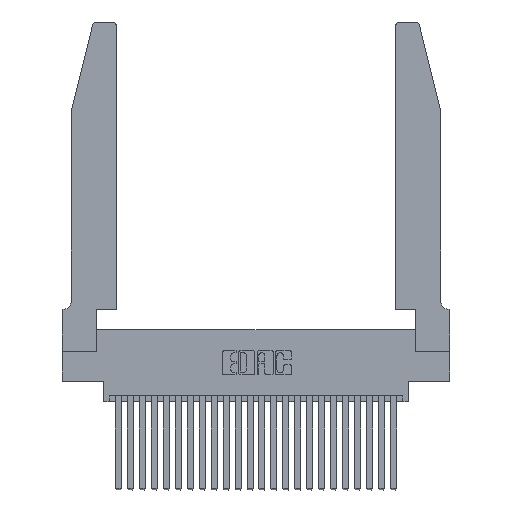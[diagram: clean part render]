
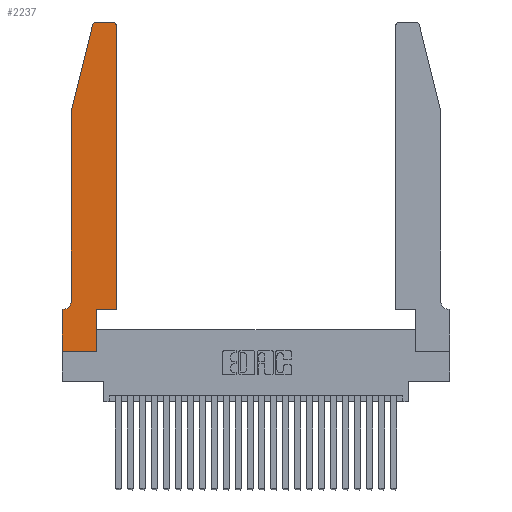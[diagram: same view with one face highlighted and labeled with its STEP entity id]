
A CAD part, top view. The second image highlights one B-rep face of the part: STEP entity #2237.
In plain terms, the highlighted planar face has unit normal (0, 0, 1).
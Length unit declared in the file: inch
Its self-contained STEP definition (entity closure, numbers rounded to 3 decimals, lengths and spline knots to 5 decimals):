
#209 = DIRECTION ( 'NONE',  ( 0., -1., 0. ) ) ;
#826 = PLANE ( 'NONE',  #3840 ) ;
#940 = DIRECTION ( 'NONE',  ( 1., 0., 0. ) ) ;
#1309 = VECTOR ( 'NONE', #20202, 39.37008 ) ;
#1359 = ORIENTED_EDGE ( 'NONE', *, *, #10340, .T. ) ;
#1753 = CARTESIAN_POINT ( 'NONE',  ( 0., 0.35, 0.37 ) ) ;
#2237 = ADVANCED_FACE ( 'NONE', ( #5001 ), #826, .T. ) ;
#2277 = DIRECTION ( 'NONE',  ( 0., 0., -1. ) ) ;
#2393 = AXIS2_PLACEMENT_3D ( 'NONE', #6460, #20418, #8505 ) ;
#2628 = EDGE_CURVE ( 'NONE', #16417, #22275, #22827, .T. ) ;
#2946 = EDGE_CURVE ( 'NONE', #23687, #5121, #10706, .T. ) ;
#3197 = CARTESIAN_POINT ( 'NONE',  ( 0., 0., 0.37 ) ) ;
#3604 = EDGE_CURVE ( 'NONE', #17030, #17161, #9738, .T. ) ;
#3840 = AXIS2_PLACEMENT_3D ( 'NONE', #1753, #6134, #940 ) ;
#3961 = VERTEX_POINT ( 'NONE', #18576 ) ;
#4518 = CIRCLE ( 'NONE', #2393, 0.03 ) ;
#4694 = CARTESIAN_POINT ( 'NONE',  ( 0.0055, 0.35, 0.37 ) ) ;
#5001 = FACE_OUTER_BOUND ( 'NONE', #18183, .T. ) ;
#5083 = VERTEX_POINT ( 'NONE', #9892 ) ;
#5121 = VERTEX_POINT ( 'NONE', #12223 ) ;
#6134 = DIRECTION ( 'NONE',  ( 0., 0., 1. ) ) ;
#6165 = CARTESIAN_POINT ( 'NONE',  ( 0.0755, 2., 0.37 ) ) ;
#6253 = CARTESIAN_POINT ( 'NONE',  ( 0.0755, 0.35, 0.37 ) ) ;
#6460 = CARTESIAN_POINT ( 'NONE',  ( 0.4205, 2.72, 0.37 ) ) ;
#6468 = CARTESIAN_POINT ( 'NONE',  ( 0., 0., 0.37 ) ) ;
#6671 = VERTEX_POINT ( 'NONE', #7288 ) ;
#7288 = CARTESIAN_POINT ( 'NONE',  ( 0.284, 2.75, 0.37 ) ) ;
#7772 = LINE ( 'NONE', #3197, #18314 ) ;
#7839 = DIRECTION ( 'NONE',  ( -0.239, -0.971, 0. ) ) ;
#7926 = CARTESIAN_POINT ( 'NONE',  ( 0.0755, 2., 0.37 ) ) ;
#8374 = LINE ( 'NONE', #21197, #14330 ) ;
#8505 = DIRECTION ( 'NONE',  ( 1., 0., 0. ) ) ;
#8970 = EDGE_CURVE ( 'NONE', #11665, #22641, #4518, .T. ) ;
#9226 = DIRECTION ( 'NONE',  ( 0., 1., 0. ) ) ;
#9245 = EDGE_CURVE ( 'NONE', #17161, #3961, #8374, .T. ) ;
#9275 = EDGE_CURVE ( 'NONE', #5121, #17030, #7772, .T. ) ;
#9416 = DIRECTION ( 'NONE',  ( 0., 1., 0. ) ) ;
#9455 = LINE ( 'NONE', #17042, #19396 ) ;
#9573 = EDGE_CURVE ( 'NONE', #24783, #23687, #22062, .T. ) ;
#9678 = CARTESIAN_POINT ( 'NONE',  ( 0.4205, 2.75, 0.37 ) ) ;
#9738 = LINE ( 'NONE', #23306, #24909 ) ;
#9810 = ORIENTED_EDGE ( 'NONE', *, *, #23884, .T. ) ;
#9892 = CARTESIAN_POINT ( 'NONE',  ( 0.25487, 2.72718, 0.37 ) ) ;
#9903 = VECTOR ( 'NONE', #9226, 39.37008 ) ;
#10340 = EDGE_CURVE ( 'NONE', #3961, #11665, #22327, .T. ) ;
#10706 = LINE ( 'NONE', #6468, #20649 ) ;
#11363 = ORIENTED_EDGE ( 'NONE', *, *, #24222, .T. ) ;
#11665 = VERTEX_POINT ( 'NONE', #19056 ) ;
#11939 = CARTESIAN_POINT ( 'NONE',  ( 0.284, 2.72, 0.37 ) ) ;
#12223 = CARTESIAN_POINT ( 'NONE',  ( 0., 0., 0.37 ) ) ;
#12286 = VECTOR ( 'NONE', #209, 39.37008 ) ;
#12428 = ORIENTED_EDGE ( 'NONE', *, *, #2628, .T. ) ;
#13769 = AXIS2_PLACEMENT_3D ( 'NONE', #14412, #2277, #16413 ) ;
#13965 = DIRECTION ( 'NONE',  ( 1., 0., 0. ) ) ;
#14162 = CARTESIAN_POINT ( 'NONE',  ( 0.0755, 0.42, 0.37 ) ) ;
#14224 = VECTOR ( 'NONE', #7839, 39.37008 ) ;
#14330 = VECTOR ( 'NONE', #19084, 39.37008 ) ;
#14412 = CARTESIAN_POINT ( 'NONE',  ( 0.0055, 0.42, 0.37 ) ) ;
#14888 = CIRCLE ( 'NONE', #13769, 0.07 ) ;
#15319 = DIRECTION ( 'NONE',  ( 1., 0., 0. ) ) ;
#15798 = ORIENTED_EDGE ( 'NONE', *, *, #3604, .T. ) ;
#16300 = ORIENTED_EDGE ( 'NONE', *, *, #9275, .T. ) ;
#16413 = DIRECTION ( 'NONE',  ( -1., 0., 0. ) ) ;
#16417 = VERTEX_POINT ( 'NONE', #24632 ) ;
#16837 = CARTESIAN_POINT ( 'NONE',  ( 0.2865, 0., 0.37 ) ) ;
#16944 = CIRCLE ( 'NONE', #25110, 0.03 ) ;
#16961 = ORIENTED_EDGE ( 'NONE', *, *, #9573, .T. ) ;
#17030 = VERTEX_POINT ( 'NONE', #16837 ) ;
#17042 = CARTESIAN_POINT ( 'NONE',  ( 0.2605, 2.75, 0.37 ) ) ;
#17161 = VERTEX_POINT ( 'NONE', #23163 ) ;
#17481 = ORIENTED_EDGE ( 'NONE', *, *, #18728, .T. ) ;
#17767 = EDGE_CURVE ( 'NONE', #22275, #24783, #14888, .T. ) ;
#18183 = EDGE_LOOP ( 'NONE', ( #11363, #9810, #17481, #12428, #21734, #16961, #18299, #16300, #15798, #21593, #1359, #25187 ) ) ;
#18299 = ORIENTED_EDGE ( 'NONE', *, *, #2946, .T. ) ;
#18314 = VECTOR ( 'NONE', #15319, 39.37008 ) ;
#18576 = CARTESIAN_POINT ( 'NONE',  ( 0.4505, 0.35, 0.37 ) ) ;
#18728 = EDGE_CURVE ( 'NONE', #5083, #16417, #24106, .T. ) ;
#19002 = DIRECTION ( 'NONE',  ( -1., 0., 0. ) ) ;
#19056 = CARTESIAN_POINT ( 'NONE',  ( 0.4505, 2.72, 0.37 ) ) ;
#19084 = DIRECTION ( 'NONE',  ( 1., 0., 0. ) ) ;
#19396 = VECTOR ( 'NONE', #19002, 39.37008 ) ;
#20202 = DIRECTION ( 'NONE',  ( -1., 0., 0. ) ) ;
#20418 = DIRECTION ( 'NONE',  ( 0., 0., 1. ) ) ;
#20649 = VECTOR ( 'NONE', #22418, 39.37008 ) ;
#21197 = CARTESIAN_POINT ( 'NONE',  ( 0.4505, 0.35, 0.37 ) ) ;
#21593 = ORIENTED_EDGE ( 'NONE', *, *, #9245, .T. ) ;
#21734 = ORIENTED_EDGE ( 'NONE', *, *, #17767, .T. ) ;
#22062 = LINE ( 'NONE', #6253, #1309 ) ;
#22275 = VERTEX_POINT ( 'NONE', #14162 ) ;
#22327 = LINE ( 'NONE', #23040, #9903 ) ;
#22418 = DIRECTION ( 'NONE',  ( 0., -1., 0. ) ) ;
#22641 = VERTEX_POINT ( 'NONE', #9678 ) ;
#22827 = LINE ( 'NONE', #6165, #12286 ) ;
#23040 = CARTESIAN_POINT ( 'NONE',  ( 0.4505, 0.35, 0.37 ) ) ;
#23163 = CARTESIAN_POINT ( 'NONE',  ( 0.2865, 0.35, 0.37 ) ) ;
#23306 = CARTESIAN_POINT ( 'NONE',  ( 0.2865, 0.35, 0.37 ) ) ;
#23687 = VERTEX_POINT ( 'NONE', #25101 ) ;
#23884 = EDGE_CURVE ( 'NONE', #6671, #5083, #16944, .T. ) ;
#24106 = LINE ( 'NONE', #7926, #14224 ) ;
#24222 = EDGE_CURVE ( 'NONE', #22641, #6671, #9455, .T. ) ;
#24632 = CARTESIAN_POINT ( 'NONE',  ( 0.0755, 2., 0.37 ) ) ;
#24783 = VERTEX_POINT ( 'NONE', #4694 ) ;
#24909 = VECTOR ( 'NONE', #9416, 39.37008 ) ;
#25101 = CARTESIAN_POINT ( 'NONE',  ( 0., 0.35, 0.37 ) ) ;
#25110 = AXIS2_PLACEMENT_3D ( 'NONE', #11939, #25794, #13965 ) ;
#25187 = ORIENTED_EDGE ( 'NONE', *, *, #8970, .T. ) ;
#25794 = DIRECTION ( 'NONE',  ( 0., 0., 1. ) ) ;
